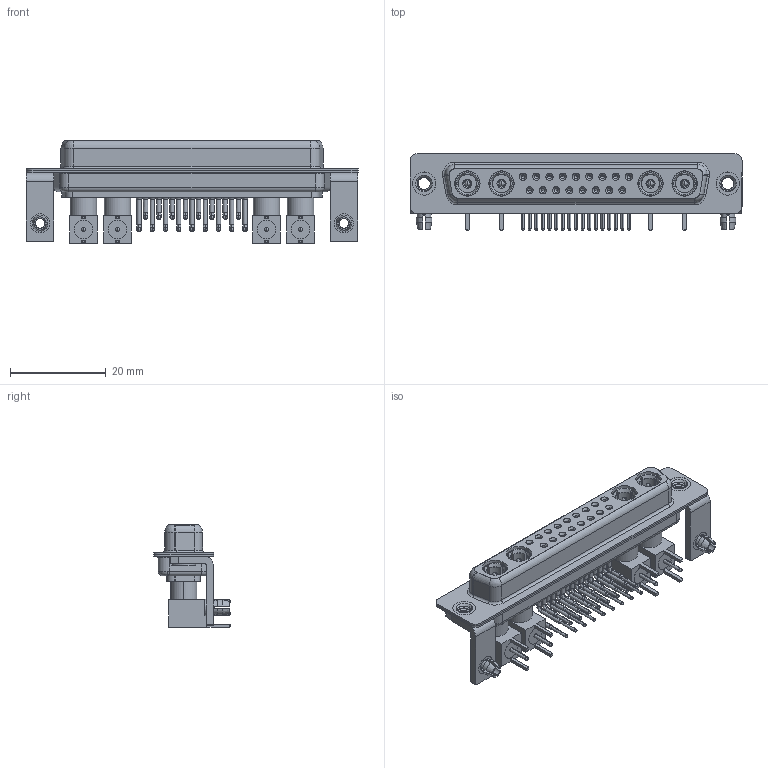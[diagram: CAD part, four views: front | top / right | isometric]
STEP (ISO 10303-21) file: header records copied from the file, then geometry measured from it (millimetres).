
FILE_DESCRIPTION (( 'STEP AP203' ), '1' );
FILE_NAME ('630-21W4640-5NB.STEP', '2022-06-08T18:50:05', ( '' ), ( '' ), 'SwSTEP 2.0', 'SolidWorks 2020', '' );
FILE_SCHEMA (( 'CONFIG_CONTROL_DESIGN' ));
Length unit declared in the file: millimetre
Products named in the file (19): Co-Ax Plug Assy_RA; 630Combo Stabilizer Bracket; 630Combo Contact Row 1; 630Combo Shell Rear_37 Contacts; 630Combo Threaded Rivet_B; Pin_RA; Insulator Pin_Straight PC Tail; RA Back Shell; 630Combo Housing_21W4; 630Combo Contact Row 2; 630Combo Board Lock; 630Combo Shell Front_37 Contacts; 630-21W4640-5NB; Co-Ax Plug_RA PC Tail; Locking Collar; Insulator RA Pin
Assembly tree (54 placements, depth 3):
  630-21W4640-5NB
    630Combo Housing_21W4
    630Combo Shell Front_37 Contacts
    630Combo Shell Rear_37 Contacts
    630Combo Threaded Rivet_B  x2
    630Combo Stabilizer Bracket  x2
    630Combo Board Lock  x2
    Co-Ax Plug Assy_RA
      Co-Ax Plug_RA PC Tail
      Insulator Pin_Straight PC Tail
      Pin_RA
      Locking Collar
      RA Back Shell
      Insulator RA Pin
    Co-Ax Plug Assy_RA
      Co-Ax Plug_RA PC Tail
      Insulator Pin_Straight PC Tail
      Pin_RA
      Locking Collar
      RA Back Shell
      Insulator RA Pin
    Co-Ax Plug Assy_RA
      Co-Ax Plug_RA PC Tail
      Insulator Pin_Straight PC Tail
      Pin_RA
      Locking Collar
      RA Back Shell
      Insulator RA Pin
    Co-Ax Plug Assy_RA
      Co-Ax Plug_RA PC Tail
      Insulator Pin_Straight PC Tail
      Pin_RA
      Locking Collar
      RA Back Shell
      Insulator RA Pin
    630Combo Contact Row 1  x9
    630Combo Contact Row 2  x8
Bounding box: 69.4 x 16 x 21.41 mm (x, y, z)
Volume: 6637.6 mm3; surface area: 15842.1 mm2
Topology: 50 solids, 50 shells, 1982 faces, 4928 edges, 3102 vertices
Faces by surface type: cylinder 838, plane 658, cone 311, torus 81, bspline 78, sphere 16
Entity records: 28257 total; most frequent: CARTESIAN_POINT 5999, DIRECTION 4421, ORIENTED_EDGE 3766, EDGE_CURVE 1883, AXIS2_PLACEMENT_3D 1813, VERTEX_POINT 1201, CIRCLE 969, EDGE_LOOP 950
